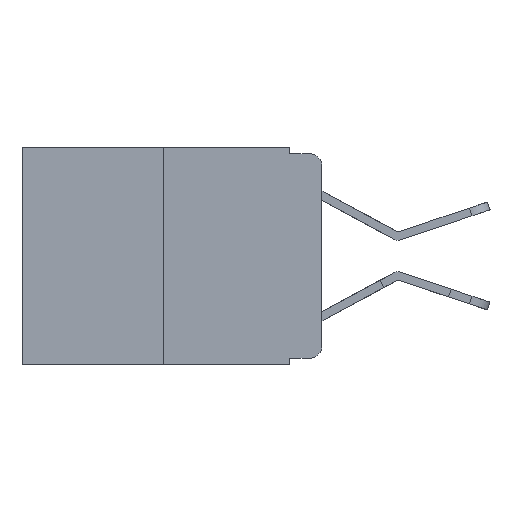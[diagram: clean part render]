
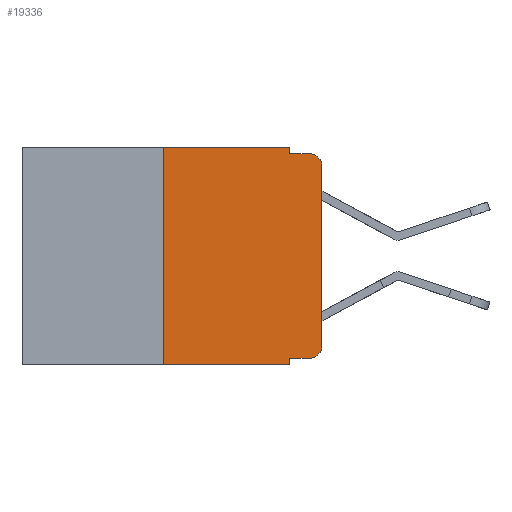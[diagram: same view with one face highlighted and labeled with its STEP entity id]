
A CAD part, left-side view. The second image highlights one B-rep face of the part: STEP entity #19336.
In plain terms, the highlighted planar face has unit normal (-1, 0, 0).
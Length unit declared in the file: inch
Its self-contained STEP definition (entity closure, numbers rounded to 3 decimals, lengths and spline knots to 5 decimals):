
#121 = CARTESIAN_POINT ( 'NONE',  ( 0., 0.25, 0. ) ) ;
#257 = DIRECTION ( 'NONE',  ( 0., -1., 0. ) ) ;
#297 = LINE ( 'NONE', #9682, #9907 ) ;
#306 = DIRECTION ( 'NONE',  ( 0., 0., -1. ) ) ;
#391 = EDGE_CURVE ( 'NONE', #21983, #20589, #13786, .T. ) ;
#531 = LINE ( 'NONE', #18570, #10761 ) ;
#561 = EDGE_CURVE ( 'NONE', #20928, #17202, #19940, .T. ) ;
#564 = PLANE ( 'NONE',  #11545 ) ;
#1563 = CARTESIAN_POINT ( 'NONE',  ( 0., 0.25, -0.343 ) ) ;
#2268 = DIRECTION ( 'NONE',  ( -1., 0., 0. ) ) ;
#2751 = DIRECTION ( 'NONE',  ( 0., 0., -1. ) ) ;
#2765 = EDGE_CURVE ( 'NONE', #3855, #20474, #297, .T. ) ;
#2799 = AXIS2_PLACEMENT_3D ( 'NONE', #23110, #20734, #7083 ) ;
#2966 = CARTESIAN_POINT ( 'NONE',  ( 0., 0.02, -0.333 ) ) ;
#3038 = FACE_OUTER_BOUND ( 'NONE', #10418, .T. ) ;
#3087 = VECTOR ( 'NONE', #306, 39.37008 ) ;
#3200 = VECTOR ( 'NONE', #25401, 39.37008 ) ;
#3732 = EDGE_CURVE ( 'NONE', #20474, #10330, #24449, .T. ) ;
#3855 = VERTEX_POINT ( 'NONE', #15461 ) ;
#3924 = ORIENTED_EDGE ( 'NONE', *, *, #561, .T. ) ;
#3972 = EDGE_CURVE ( 'NONE', #17202, #3855, #14255, .T. ) ;
#4152 = CARTESIAN_POINT ( 'NONE',  ( 0., 0.051, 0. ) ) ;
#4165 = DIRECTION ( 'NONE',  ( 0., 0., -1. ) ) ;
#4902 = DIRECTION ( 'NONE',  ( 0., 0., -1. ) ) ;
#4905 = DIRECTION ( 'NONE',  ( 0., -1., 0. ) ) ;
#5167 = EDGE_CURVE ( 'NONE', #20173, #22717, #19145, .T. ) ;
#5219 = LINE ( 'NONE', #14141, #9875 ) ;
#6900 = CARTESIAN_POINT ( 'NONE',  ( 0., 0.051, -0.01 ) ) ;
#6902 = CARTESIAN_POINT ( 'NONE',  ( 0., 0.051, -0.333 ) ) ;
#7083 = DIRECTION ( 'NONE',  ( 0., 0., -1. ) ) ;
#7441 = EDGE_CURVE ( 'NONE', #20173, #18166, #531, .T. ) ;
#7723 = LINE ( 'NONE', #8541, #11788 ) ;
#8164 = CARTESIAN_POINT ( 'NONE',  ( 0., 0.25, 0. ) ) ;
#8541 = CARTESIAN_POINT ( 'NONE',  ( 0., 0.473, 0. ) ) ;
#8616 = DIRECTION ( 'NONE',  ( 0., -1., 0. ) ) ;
#9314 = DIRECTION ( 'NONE',  ( 0., -1., 0. ) ) ;
#9351 = VECTOR ( 'NONE', #9314, 39.37008 ) ;
#9682 = CARTESIAN_POINT ( 'NONE',  ( 0., 0., 0. ) ) ;
#9875 = VECTOR ( 'NONE', #4165, 39.37008 ) ;
#9907 = VECTOR ( 'NONE', #10976, 39.37008 ) ;
#10330 = VERTEX_POINT ( 'NONE', #14732 ) ;
#10366 = AXIS2_PLACEMENT_3D ( 'NONE', #10657, #2268, #4902 ) ;
#10418 = EDGE_LOOP ( 'NONE', ( #23718, #24448, #24156, #25071, #25285, #23508, #25339, #18623, #3924, #12215 ) ) ;
#10657 = CARTESIAN_POINT ( 'NONE',  ( 0., 0.02, -0.313 ) ) ;
#10743 = CARTESIAN_POINT ( 'NONE',  ( 0., 0.473, 0. ) ) ;
#10761 = VECTOR ( 'NONE', #8616, 39.37008 ) ;
#10976 = DIRECTION ( 'NONE',  ( 0., 0., 1. ) ) ;
#11545 = AXIS2_PLACEMENT_3D ( 'NONE', #10743, #14787, #2751 ) ;
#11788 = VECTOR ( 'NONE', #257, 39.37008 ) ;
#12215 = ORIENTED_EDGE ( 'NONE', *, *, #3972, .T. ) ;
#13786 = LINE ( 'NONE', #4152, #3087 ) ;
#14141 = CARTESIAN_POINT ( 'NONE',  ( 0., 0.051, 0. ) ) ;
#14255 = CIRCLE ( 'NONE', #10366, 0.02 ) ;
#14542 = EDGE_CURVE ( 'NONE', #20589, #10330, #16292, .T. ) ;
#14732 = CARTESIAN_POINT ( 'NONE',  ( 0., 0.02, -0.01 ) ) ;
#14778 = CARTESIAN_POINT ( 'NONE',  ( 0., 0., -0.03 ) ) ;
#14787 = DIRECTION ( 'NONE',  ( 1., 0., 0. ) ) ;
#15461 = CARTESIAN_POINT ( 'NONE',  ( 0., 0., -0.313 ) ) ;
#15958 = CARTESIAN_POINT ( 'NONE',  ( 0., 0.051, -0.343 ) ) ;
#16292 = LINE ( 'NONE', #6900, #20909 ) ;
#17202 = VERTEX_POINT ( 'NONE', #2966 ) ;
#18166 = VERTEX_POINT ( 'NONE', #15958 ) ;
#18570 = CARTESIAN_POINT ( 'NONE',  ( 0., 0.473, -0.343 ) ) ;
#18623 = ORIENTED_EDGE ( 'NONE', *, *, #20316, .F. ) ;
#19145 = LINE ( 'NONE', #121, #3200 ) ;
#19336 = ADVANCED_FACE ( 'NONE', ( #3038 ), #564, .F. ) ;
#19784 = EDGE_CURVE ( 'NONE', #22717, #21983, #7723, .T. ) ;
#19940 = LINE ( 'NONE', #6902, #9351 ) ;
#20173 = VERTEX_POINT ( 'NONE', #1563 ) ;
#20316 = EDGE_CURVE ( 'NONE', #20928, #18166, #5219, .T. ) ;
#20474 = VERTEX_POINT ( 'NONE', #14778 ) ;
#20589 = VERTEX_POINT ( 'NONE', #23115 ) ;
#20734 = DIRECTION ( 'NONE',  ( -1., 0., 0. ) ) ;
#20909 = VECTOR ( 'NONE', #4905, 39.37008 ) ;
#20928 = VERTEX_POINT ( 'NONE', #22597 ) ;
#21983 = VERTEX_POINT ( 'NONE', #25265 ) ;
#22597 = CARTESIAN_POINT ( 'NONE',  ( 0., 0.051, -0.333 ) ) ;
#22717 = VERTEX_POINT ( 'NONE', #8164 ) ;
#23110 = CARTESIAN_POINT ( 'NONE',  ( 0., 0.02, -0.03 ) ) ;
#23115 = CARTESIAN_POINT ( 'NONE',  ( 0., 0.051, -0.01 ) ) ;
#23508 = ORIENTED_EDGE ( 'NONE', *, *, #5167, .F. ) ;
#23718 = ORIENTED_EDGE ( 'NONE', *, *, #2765, .T. ) ;
#24156 = ORIENTED_EDGE ( 'NONE', *, *, #14542, .F. ) ;
#24448 = ORIENTED_EDGE ( 'NONE', *, *, #3732, .T. ) ;
#24449 = CIRCLE ( 'NONE', #2799, 0.02 ) ;
#25071 = ORIENTED_EDGE ( 'NONE', *, *, #391, .F. ) ;
#25265 = CARTESIAN_POINT ( 'NONE',  ( 0., 0.051, 0. ) ) ;
#25285 = ORIENTED_EDGE ( 'NONE', *, *, #19784, .F. ) ;
#25339 = ORIENTED_EDGE ( 'NONE', *, *, #7441, .T. ) ;
#25401 = DIRECTION ( 'NONE',  ( 0., 0., 1. ) ) ;
